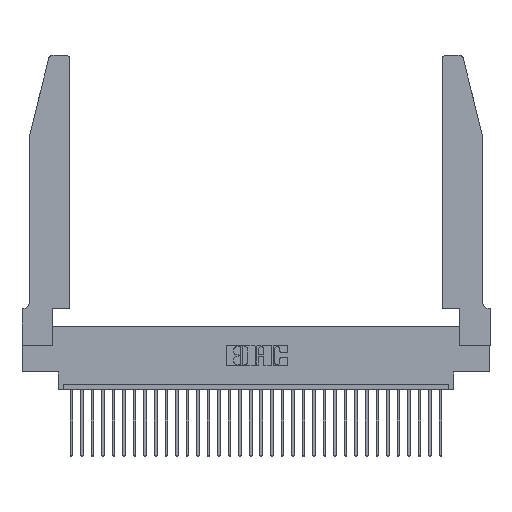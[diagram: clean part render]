
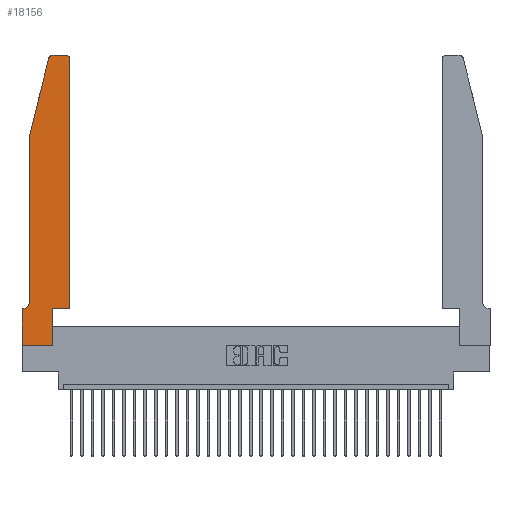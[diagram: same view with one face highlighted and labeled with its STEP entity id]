
A CAD part, top view. The second image highlights one B-rep face of the part: STEP entity #18156.
In plain terms, the highlighted planar face has unit normal (0, 0, 1).
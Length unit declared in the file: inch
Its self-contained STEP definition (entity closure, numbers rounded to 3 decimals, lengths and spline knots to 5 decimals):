
#323 = VECTOR ( 'NONE', #24473, 39.37008 ) ;
#492 = VECTOR ( 'NONE', #5316, 39.37008 ) ;
#708 = VECTOR ( 'NONE', #14088, 39.37008 ) ;
#740 = CARTESIAN_POINT ( 'NONE',  ( 0.284, 2.75, 0.37 ) ) ;
#753 = ORIENTED_EDGE ( 'NONE', *, *, #13437, .T. ) ;
#865 = DIRECTION ( 'NONE',  ( -0.239, -0.971, 0. ) ) ;
#1088 = EDGE_CURVE ( 'NONE', #28173, #20522, #23746, .T. ) ;
#1314 = DIRECTION ( 'NONE',  ( -1., 0., 0. ) ) ;
#1616 = DIRECTION ( 'NONE',  ( 0., 0., -1. ) ) ;
#1686 = VERTEX_POINT ( 'NONE', #740 ) ;
#2104 = DIRECTION ( 'NONE',  ( 0., 0., 1. ) ) ;
#2694 = AXIS2_PLACEMENT_3D ( 'NONE', #5035, #12321, #14841 ) ;
#2736 = ORIENTED_EDGE ( 'NONE', *, *, #22850, .T. ) ;
#3059 = ORIENTED_EDGE ( 'NONE', *, *, #1088, .T. ) ;
#4411 = CARTESIAN_POINT ( 'NONE',  ( 0.0055, 0.42, 0.37 ) ) ;
#4432 = LINE ( 'NONE', #14947, #14400 ) ;
#4858 = VECTOR ( 'NONE', #10313, 39.37008 ) ;
#5035 = CARTESIAN_POINT ( 'NONE',  ( 0., 0.35, 0.37 ) ) ;
#5159 = EDGE_CURVE ( 'NONE', #16437, #15930, #21924, .T. ) ;
#5252 = VERTEX_POINT ( 'NONE', #29139 ) ;
#5316 = DIRECTION ( 'NONE',  ( 1., 0., 0. ) ) ;
#5855 = CARTESIAN_POINT ( 'NONE',  ( 0.0755, 2., 0.37 ) ) ;
#6047 = FACE_OUTER_BOUND ( 'NONE', #14561, .T. ) ;
#6855 = VERTEX_POINT ( 'NONE', #30363 ) ;
#7216 = VERTEX_POINT ( 'NONE', #25928 ) ;
#7298 = VECTOR ( 'NONE', #28823, 39.37008 ) ;
#7334 = CARTESIAN_POINT ( 'NONE',  ( 0.0755, 0.35, 0.37 ) ) ;
#7347 = CARTESIAN_POINT ( 'NONE',  ( 0.4505, 2.72, 0.37 ) ) ;
#7888 = CARTESIAN_POINT ( 'NONE',  ( 0.2865, 0.35, 0.37 ) ) ;
#8262 = ORIENTED_EDGE ( 'NONE', *, *, #18118, .T. ) ;
#8566 = DIRECTION ( 'NONE',  ( 1., 0., 0. ) ) ;
#8671 = EDGE_CURVE ( 'NONE', #20522, #15223, #15853, .T. ) ;
#8746 = LINE ( 'NONE', #19279, #323 ) ;
#9695 = DIRECTION ( 'NONE',  ( -1., 0., 0. ) ) ;
#9718 = AXIS2_PLACEMENT_3D ( 'NONE', #16225, #21208, #13469 ) ;
#10313 = DIRECTION ( 'NONE',  ( -1., 0., 0. ) ) ;
#10437 = ORIENTED_EDGE ( 'NONE', *, *, #5159, .T. ) ;
#10528 = EDGE_CURVE ( 'NONE', #14847, #1686, #24449, .T. ) ;
#10566 = CARTESIAN_POINT ( 'NONE',  ( 0., 0., 0.37 ) ) ;
#11833 = CIRCLE ( 'NONE', #31228, 0.03 ) ;
#12321 = DIRECTION ( 'NONE',  ( 0., 0., 1. ) ) ;
#13437 = EDGE_CURVE ( 'NONE', #6855, #30516, #15473, .T. ) ;
#13469 = DIRECTION ( 'NONE',  ( 1., 0., 0. ) ) ;
#13649 = CARTESIAN_POINT ( 'NONE',  ( 0.0755, 2., 0.37 ) ) ;
#14088 = DIRECTION ( 'NONE',  ( 0., 1., 0. ) ) ;
#14400 = VECTOR ( 'NONE', #30254, 39.37008 ) ;
#14485 = CARTESIAN_POINT ( 'NONE',  ( 0.2865, 0.35, 0.37 ) ) ;
#14561 = EDGE_LOOP ( 'NONE', ( #32570, #18065, #753, #23239, #24699, #10437, #2736, #3059, #19789, #22319, #8262, #23294 ) ) ;
#14757 = EDGE_CURVE ( 'NONE', #30853, #14847, #11833, .T. ) ;
#14841 = DIRECTION ( 'NONE',  ( 1., 0., 0. ) ) ;
#14847 = VERTEX_POINT ( 'NONE', #29896 ) ;
#14947 = CARTESIAN_POINT ( 'NONE',  ( 0.4505, 0.35, 0.37 ) ) ;
#15016 = EDGE_CURVE ( 'NONE', #1686, #6855, #16950, .T. ) ;
#15223 = VERTEX_POINT ( 'NONE', #7888 ) ;
#15473 = LINE ( 'NONE', #24096, #32449 ) ;
#15853 = LINE ( 'NONE', #14485, #708 ) ;
#15930 = VERTEX_POINT ( 'NONE', #29816 ) ;
#16225 = CARTESIAN_POINT ( 'NONE',  ( 0.284, 2.72, 0.37 ) ) ;
#16437 = VERTEX_POINT ( 'NONE', #19633 ) ;
#16950 = CIRCLE ( 'NONE', #9718, 0.03 ) ;
#18028 = EDGE_CURVE ( 'NONE', #30516, #7216, #24718, .T. ) ;
#18065 = ORIENTED_EDGE ( 'NONE', *, *, #15016, .T. ) ;
#18080 = CARTESIAN_POINT ( 'NONE',  ( 0.4205, 2.72, 0.37 ) ) ;
#18118 = EDGE_CURVE ( 'NONE', #5252, #30853, #4432, .T. ) ;
#18156 = ADVANCED_FACE ( 'NONE', ( #6047 ), #20033, .T. ) ;
#19279 = CARTESIAN_POINT ( 'NONE',  ( 0., 0., 0.37 ) ) ;
#19633 = CARTESIAN_POINT ( 'NONE',  ( 0.0055, 0.35, 0.37 ) ) ;
#19789 = ORIENTED_EDGE ( 'NONE', *, *, #8671, .T. ) ;
#20033 = PLANE ( 'NONE',  #2694 ) ;
#20148 = CARTESIAN_POINT ( 'NONE',  ( 0., 0., 0.37 ) ) ;
#20522 = VERTEX_POINT ( 'NONE', #25838 ) ;
#21208 = DIRECTION ( 'NONE',  ( 0., 0., 1. ) ) ;
#21924 = LINE ( 'NONE', #7334, #4858 ) ;
#22319 = ORIENTED_EDGE ( 'NONE', *, *, #32048, .T. ) ;
#22610 = VECTOR ( 'NONE', #25588, 39.37008 ) ;
#22850 = EDGE_CURVE ( 'NONE', #15930, #28173, #8746, .T. ) ;
#23239 = ORIENTED_EDGE ( 'NONE', *, *, #18028, .T. ) ;
#23294 = ORIENTED_EDGE ( 'NONE', *, *, #14757, .T. ) ;
#23746 = LINE ( 'NONE', #10566, #22610 ) ;
#24096 = CARTESIAN_POINT ( 'NONE',  ( 0.0755, 2., 0.37 ) ) ;
#24449 = LINE ( 'NONE', #29124, #26374 ) ;
#24473 = DIRECTION ( 'NONE',  ( 0., -1., 0. ) ) ;
#24699 = ORIENTED_EDGE ( 'NONE', *, *, #28551, .T. ) ;
#24718 = LINE ( 'NONE', #5855, #7298 ) ;
#25588 = DIRECTION ( 'NONE',  ( 1., 0., 0. ) ) ;
#25838 = CARTESIAN_POINT ( 'NONE',  ( 0.2865, 0., 0.37 ) ) ;
#25928 = CARTESIAN_POINT ( 'NONE',  ( 0.0755, 0.42, 0.37 ) ) ;
#26374 = VECTOR ( 'NONE', #1314, 39.37008 ) ;
#27132 = CARTESIAN_POINT ( 'NONE',  ( 0.4505, 0.35, 0.37 ) ) ;
#27507 = LINE ( 'NONE', #27132, #492 ) ;
#28173 = VERTEX_POINT ( 'NONE', #20148 ) ;
#28551 = EDGE_CURVE ( 'NONE', #7216, #16437, #31953, .T. ) ;
#28823 = DIRECTION ( 'NONE',  ( 0., -1., 0. ) ) ;
#29124 = CARTESIAN_POINT ( 'NONE',  ( 0.2605, 2.75, 0.37 ) ) ;
#29139 = CARTESIAN_POINT ( 'NONE',  ( 0.4505, 0.35, 0.37 ) ) ;
#29816 = CARTESIAN_POINT ( 'NONE',  ( 0., 0.35, 0.37 ) ) ;
#29896 = CARTESIAN_POINT ( 'NONE',  ( 0.4205, 2.75, 0.37 ) ) ;
#30254 = DIRECTION ( 'NONE',  ( 0., 1., 0. ) ) ;
#30363 = CARTESIAN_POINT ( 'NONE',  ( 0.25487, 2.72718, 0.37 ) ) ;
#30516 = VERTEX_POINT ( 'NONE', #13649 ) ;
#30853 = VERTEX_POINT ( 'NONE', #7347 ) ;
#31228 = AXIS2_PLACEMENT_3D ( 'NONE', #18080, #2104, #8566 ) ;
#31699 = AXIS2_PLACEMENT_3D ( 'NONE', #4411, #1616, #9695 ) ;
#31953 = CIRCLE ( 'NONE', #31699, 0.07 ) ;
#32048 = EDGE_CURVE ( 'NONE', #15223, #5252, #27507, .T. ) ;
#32449 = VECTOR ( 'NONE', #865, 39.37008 ) ;
#32570 = ORIENTED_EDGE ( 'NONE', *, *, #10528, .T. ) ;
